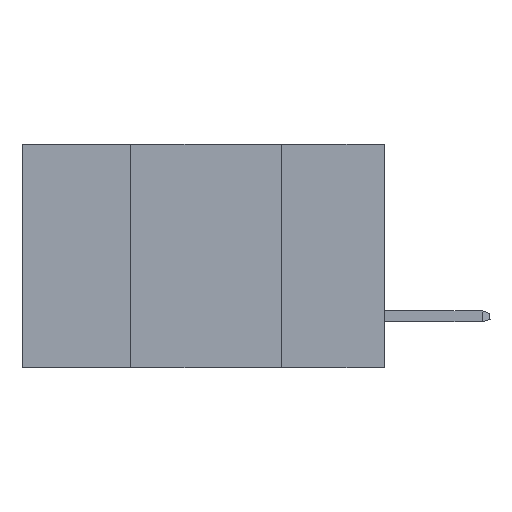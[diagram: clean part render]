
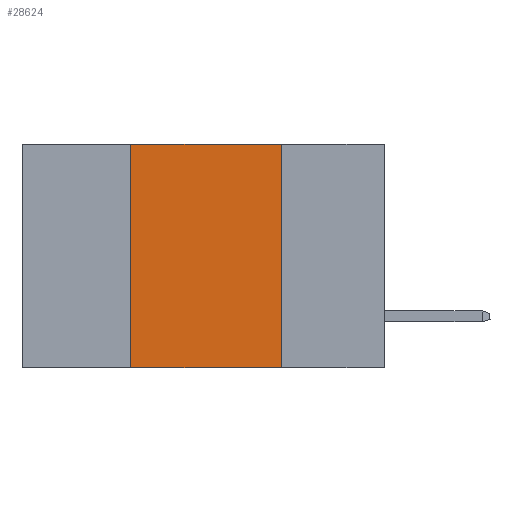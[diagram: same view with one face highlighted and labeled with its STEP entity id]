
A CAD part, left-side view. The second image highlights one B-rep face of the part: STEP entity #28624.
In plain terms, the highlighted planar face has unit normal (-1, 0, 0).
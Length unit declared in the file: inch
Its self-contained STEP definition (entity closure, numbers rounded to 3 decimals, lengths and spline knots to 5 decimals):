
#647 = FACE_OUTER_BOUND ( 'NONE', #23165, .T. ) ;
#2405 = CARTESIAN_POINT ( 'NONE',  ( 0., 0.42, 0. ) ) ;
#3463 = EDGE_CURVE ( 'NONE', #11228, #16957, #17202, .T. ) ;
#3923 = ORIENTED_EDGE ( 'NONE', *, *, #23947, .F. ) ;
#5205 = CARTESIAN_POINT ( 'NONE',  ( 0., 0.6, 0. ) ) ;
#6290 = PLANE ( 'NONE',  #17000 ) ;
#7373 = VECTOR ( 'NONE', #7587, 39.37008 ) ;
#7587 = DIRECTION ( 'NONE',  ( 0., -1., 0. ) ) ;
#8022 = CARTESIAN_POINT ( 'NONE',  ( 0., 0.17, 0. ) ) ;
#10963 = DIRECTION ( 'NONE',  ( 1., 0., 0. ) ) ;
#11228 = VERTEX_POINT ( 'NONE', #21973 ) ;
#11266 = EDGE_CURVE ( 'NONE', #26934, #14099, #20084, .T. ) ;
#12080 = DIRECTION ( 'NONE',  ( 0., 0., 1. ) ) ;
#13560 = LINE ( 'NONE', #5205, #7373 ) ;
#13764 = ORIENTED_EDGE ( 'NONE', *, *, #15610, .T. ) ;
#13921 = LINE ( 'NONE', #23370, #18772 ) ;
#14099 = VERTEX_POINT ( 'NONE', #27121 ) ;
#14200 = CARTESIAN_POINT ( 'NONE',  ( 0., 0.42, 0. ) ) ;
#15610 = EDGE_CURVE ( 'NONE', #11228, #14099, #13921, .T. ) ;
#16957 = VERTEX_POINT ( 'NONE', #14200 ) ;
#17000 = AXIS2_PLACEMENT_3D ( 'NONE', #25010, #10963, #27331 ) ;
#17202 = LINE ( 'NONE', #2405, #21969 ) ;
#18772 = VECTOR ( 'NONE', #25650, 39.37008 ) ;
#20084 = LINE ( 'NONE', #8022, #25542 ) ;
#21969 = VECTOR ( 'NONE', #12080, 39.37008 ) ;
#21973 = CARTESIAN_POINT ( 'NONE',  ( 0., 0.42, -0.37 ) ) ;
#22071 = DIRECTION ( 'NONE',  ( 0., 0., -1. ) ) ;
#22555 = ORIENTED_EDGE ( 'NONE', *, *, #3463, .F. ) ;
#23165 = EDGE_LOOP ( 'NONE', ( #23754, #3923, #22555, #13764 ) ) ;
#23370 = CARTESIAN_POINT ( 'NONE',  ( 0., 0.6, -0.37 ) ) ;
#23754 = ORIENTED_EDGE ( 'NONE', *, *, #11266, .F. ) ;
#23947 = EDGE_CURVE ( 'NONE', #16957, #26934, #13560, .T. ) ;
#25010 = CARTESIAN_POINT ( 'NONE',  ( 0., 0.6, 0. ) ) ;
#25542 = VECTOR ( 'NONE', #22071, 39.37008 ) ;
#25650 = DIRECTION ( 'NONE',  ( 0., -1., 0. ) ) ;
#26934 = VERTEX_POINT ( 'NONE', #27913 ) ;
#27121 = CARTESIAN_POINT ( 'NONE',  ( 0., 0.17, -0.37 ) ) ;
#27331 = DIRECTION ( 'NONE',  ( 0., 0., -1. ) ) ;
#27913 = CARTESIAN_POINT ( 'NONE',  ( 0., 0.17, 0. ) ) ;
#28624 = ADVANCED_FACE ( 'NONE', ( #647 ), #6290, .F. ) ;
